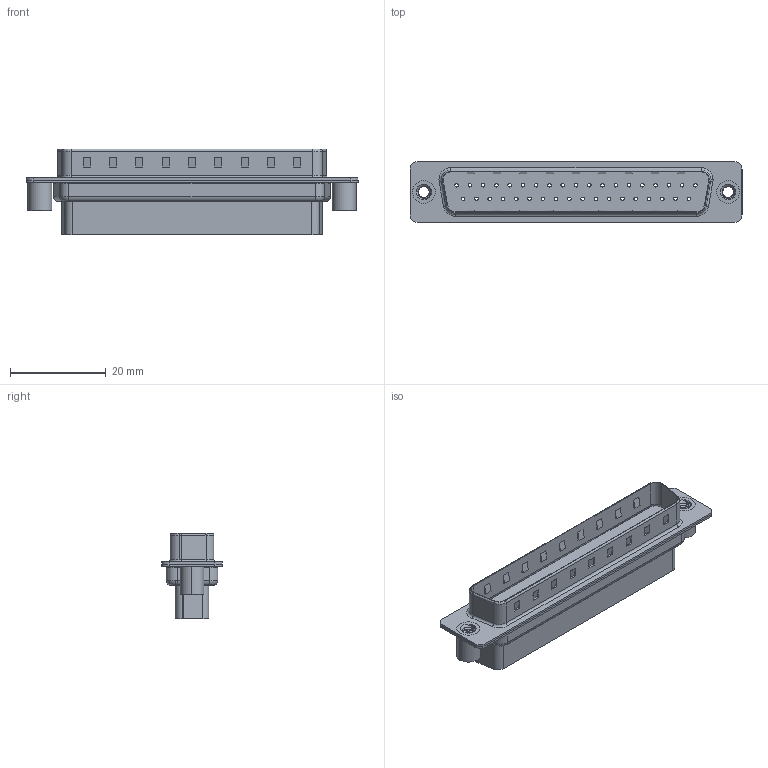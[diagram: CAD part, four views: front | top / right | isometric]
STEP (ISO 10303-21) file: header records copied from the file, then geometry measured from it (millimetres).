
FILE_DESCRIPTION (( 'STEP AP203' ), '1' );
FILE_NAME ('627-050-010-220.STEP', '2018-11-21T22:21:27', ( '' ), ( '' ), 'SwSTEP 2.0', 'SolidWorks 2016', '' );
FILE_SCHEMA (( 'CONFIG_CONTROL_DESIGN' ));
Length unit declared in the file: millimetre
Products named in the file (5): 627 4-40 Threaded Standoff BS; 627-050-010-220; 627 Housing_37 HP; 627 Shell Front_37 Contacts; 627 Shell Rear_37 Contacts
Assembly tree (5 placements, depth 2):
  627-050-010-220
    627 Housing_37 HP
    627 Shell Front_37 Contacts
    627 Shell Rear_37 Contacts
    627 4-40 Threaded Standoff BS  x2
Bounding box: 69.3 x 12.6 x 17.9 mm (x, y, z)
Volume: 5120.4 mm3; surface area: 9227.3 mm2
Topology: 5 solids, 5 shells, 730 faces, 1787 edges, 1152 vertices
Faces by surface type: cylinder 383, plane 277, torus 50, cone 14, bspline 6
Entity records: 22696 total; most frequent: CARTESIAN_POINT 5235, DIRECTION 3731, ORIENTED_EDGE 3348, EDGE_CURVE 1674, AXIS2_PLACEMENT_3D 1433, VERTEX_POINT 1079, EDGE_LOOP 893, LINE 865
